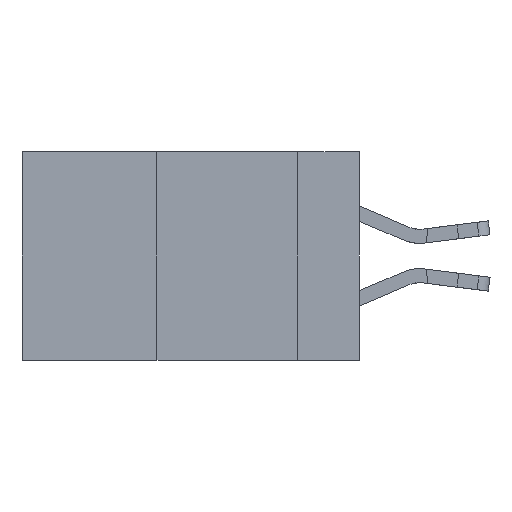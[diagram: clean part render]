
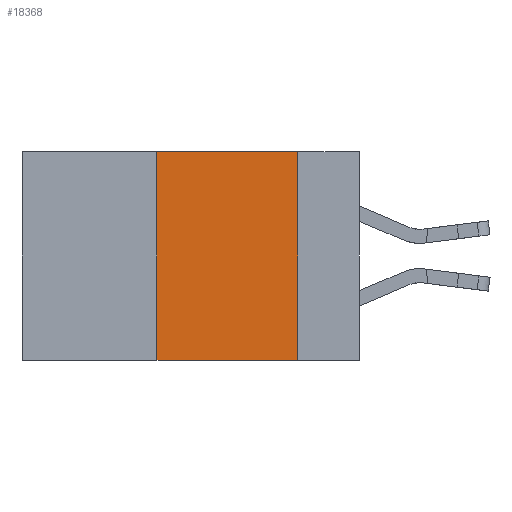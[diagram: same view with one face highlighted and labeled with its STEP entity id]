
A CAD part, left-side view. The second image highlights one B-rep face of the part: STEP entity #18368.
In plain terms, the highlighted planar face has unit normal (-1, 0, 0).
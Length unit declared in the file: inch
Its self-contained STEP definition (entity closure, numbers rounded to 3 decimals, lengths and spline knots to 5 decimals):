
#2204 = VECTOR ( 'NONE', #23622, 39.37008 ) ;
#2501 = CARTESIAN_POINT ( 'NONE',  ( 0., 0.36, -0.37 ) ) ;
#3160 = CARTESIAN_POINT ( 'NONE',  ( 0., 0.36, 0. ) ) ;
#3315 = ORIENTED_EDGE ( 'NONE', *, *, #24761, .F. ) ;
#3435 = CARTESIAN_POINT ( 'NONE',  ( 0., 0.11, -0.37 ) ) ;
#3560 = VECTOR ( 'NONE', #3993, 39.37008 ) ;
#3993 = DIRECTION ( 'NONE',  ( 0., -1., 0. ) ) ;
#4164 = VERTEX_POINT ( 'NONE', #3160 ) ;
#4484 = DIRECTION ( 'NONE',  ( 0., -1., 0. ) ) ;
#5565 = VERTEX_POINT ( 'NONE', #3435 ) ;
#5854 = CARTESIAN_POINT ( 'NONE',  ( 0., 0.6, 0. ) ) ;
#6172 = ORIENTED_EDGE ( 'NONE', *, *, #24215, .F. ) ;
#7167 = VECTOR ( 'NONE', #18909, 39.37008 ) ;
#10018 = LINE ( 'NONE', #30697, #3560 ) ;
#10622 = PLANE ( 'NONE',  #14147 ) ;
#10833 = DIRECTION ( 'NONE',  ( 1., 0., 0. ) ) ;
#11292 = VECTOR ( 'NONE', #4484, 39.37008 ) ;
#11607 = CARTESIAN_POINT ( 'NONE',  ( 0., 0.6, 0. ) ) ;
#12233 = ORIENTED_EDGE ( 'NONE', *, *, #30965, .T. ) ;
#13223 = LINE ( 'NONE', #23647, #7167 ) ;
#13771 = CARTESIAN_POINT ( 'NONE',  ( 0., 0.36, 0. ) ) ;
#14147 = AXIS2_PLACEMENT_3D ( 'NONE', #5854, #10833, #22811 ) ;
#16242 = ORIENTED_EDGE ( 'NONE', *, *, #17307, .F. ) ;
#17307 = EDGE_CURVE ( 'NONE', #26785, #5565, #13223, .T. ) ;
#18368 = ADVANCED_FACE ( 'NONE', ( #19629 ), #10622, .F. ) ;
#18549 = LINE ( 'NONE', #13771, #2204 ) ;
#18909 = DIRECTION ( 'NONE',  ( 0., 0., -1. ) ) ;
#19629 = FACE_OUTER_BOUND ( 'NONE', #20976, .T. ) ;
#20976 = EDGE_LOOP ( 'NONE', ( #16242, #3315, #6172, #12233 ) ) ;
#22811 = DIRECTION ( 'NONE',  ( 0., 0., -1. ) ) ;
#23622 = DIRECTION ( 'NONE',  ( 0., 0., 1. ) ) ;
#23647 = CARTESIAN_POINT ( 'NONE',  ( 0., 0.11, 0. ) ) ;
#24215 = EDGE_CURVE ( 'NONE', #30086, #4164, #18549, .T. ) ;
#24761 = EDGE_CURVE ( 'NONE', #4164, #26785, #24943, .T. ) ;
#24943 = LINE ( 'NONE', #11607, #11292 ) ;
#26173 = CARTESIAN_POINT ( 'NONE',  ( 0., 0.11, 0. ) ) ;
#26785 = VERTEX_POINT ( 'NONE', #26173 ) ;
#30086 = VERTEX_POINT ( 'NONE', #2501 ) ;
#30697 = CARTESIAN_POINT ( 'NONE',  ( 0., 0.6, -0.37 ) ) ;
#30965 = EDGE_CURVE ( 'NONE', #30086, #5565, #10018, .T. ) ;
